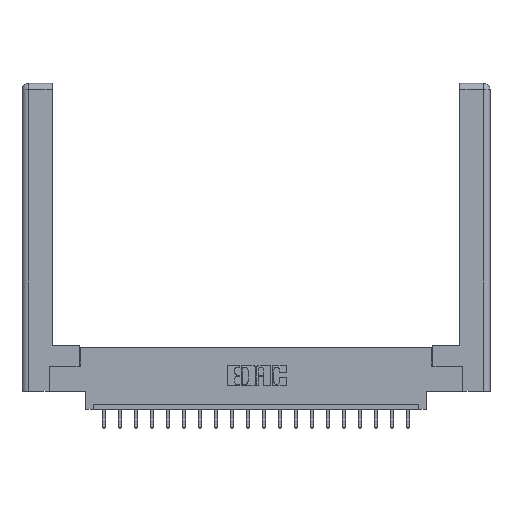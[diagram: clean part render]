
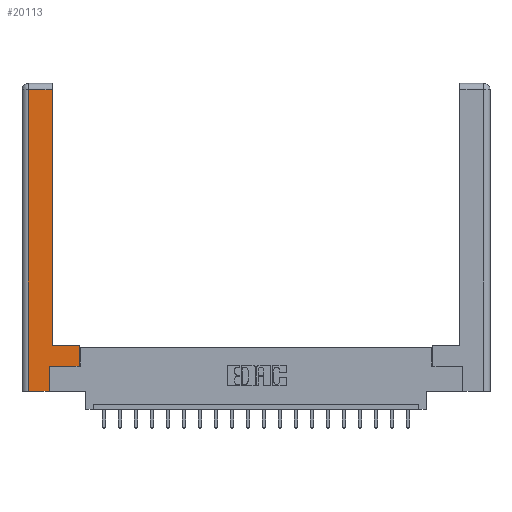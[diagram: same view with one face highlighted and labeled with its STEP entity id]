
A CAD part, top view. The second image highlights one B-rep face of the part: STEP entity #20113.
In plain terms, the highlighted planar face has unit normal (0, 0, 1).
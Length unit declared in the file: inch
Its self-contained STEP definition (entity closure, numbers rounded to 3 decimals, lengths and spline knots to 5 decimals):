
#619 = LINE ( 'NONE', #10233, #16537 ) ;
#1052 = ORIENTED_EDGE ( 'NONE', *, *, #16412, .T. ) ;
#1125 = VERTEX_POINT ( 'NONE', #10306 ) ;
#1255 = LINE ( 'NONE', #3558, #9013 ) ;
#1774 = LINE ( 'NONE', #10277, #2007 ) ;
#1930 = DIRECTION ( 'NONE',  ( 0., 1., 0. ) ) ;
#1994 = CARTESIAN_POINT ( 'NONE',  ( 0.0615, 2.94, 0. ) ) ;
#2007 = VECTOR ( 'NONE', #18453, 39.37008 ) ;
#2178 = EDGE_CURVE ( 'NONE', #15782, #13616, #1774, .T. ) ;
#2223 = ORIENTED_EDGE ( 'NONE', *, *, #10194, .T. ) ;
#2289 = CARTESIAN_POINT ( 'NONE',  ( 0.565, 0.245, 0. ) ) ;
#2512 = VECTOR ( 'NONE', #12896, 39.37008 ) ;
#3025 = DIRECTION ( 'NONE',  ( 0., 0., -1. ) ) ;
#3085 = EDGE_LOOP ( 'NONE', ( #16549, #2223, #18322, #14330, #16778, #1052, #13629, #8662 ) ) ;
#3558 = CARTESIAN_POINT ( 'NONE',  ( 0.295, 0.45, 0. ) ) ;
#3946 = DIRECTION ( 'NONE',  ( 1., 0., 0. ) ) ;
#4752 = CARTESIAN_POINT ( 'NONE',  ( 0.0615, 0., 0. ) ) ;
#5278 = CARTESIAN_POINT ( 'NONE',  ( 0.265, 0., 0. ) ) ;
#6030 = EDGE_CURVE ( 'NONE', #6105, #14938, #9864, .T. ) ;
#6105 = VERTEX_POINT ( 'NONE', #5278 ) ;
#6182 = EDGE_CURVE ( 'NONE', #7716, #6105, #619, .T. ) ;
#7032 = LINE ( 'NONE', #17950, #18241 ) ;
#7328 = CARTESIAN_POINT ( 'NONE',  ( 0.0615, 2.94, 0. ) ) ;
#7577 = EDGE_CURVE ( 'NONE', #14143, #1125, #7032, .T. ) ;
#7716 = VERTEX_POINT ( 'NONE', #18553 ) ;
#8306 = DIRECTION ( 'NONE',  ( 0., 1., 0. ) ) ;
#8662 = ORIENTED_EDGE ( 'NONE', *, *, #15277, .T. ) ;
#8668 = FACE_OUTER_BOUND ( 'NONE', #3085, .T. ) ;
#9013 = VECTOR ( 'NONE', #19487, 39.37008 ) ;
#9198 = LINE ( 'NONE', #18119, #13186 ) ;
#9386 = EDGE_CURVE ( 'NONE', #11728, #7716, #14218, .T. ) ;
#9810 = CARTESIAN_POINT ( 'NONE',  ( 0.265, 0.245, 0. ) ) ;
#9864 = LINE ( 'NONE', #9810, #18319 ) ;
#10194 = EDGE_CURVE ( 'NONE', #13616, #11728, #15916, .T. ) ;
#10233 = CARTESIAN_POINT ( 'NONE',  ( 0.265, 0., 0. ) ) ;
#10277 = CARTESIAN_POINT ( 'NONE',  ( 0.295, 3., 0. ) ) ;
#10306 = CARTESIAN_POINT ( 'NONE',  ( 0.565, 0.45, 0. ) ) ;
#10477 = VECTOR ( 'NONE', #13468, 39.37008 ) ;
#10992 = CARTESIAN_POINT ( 'NONE',  ( 0., 0., 0. ) ) ;
#11728 = VERTEX_POINT ( 'NONE', #1994 ) ;
#11969 = CARTESIAN_POINT ( 'NONE',  ( 0.295, 2.94, 0. ) ) ;
#12896 = DIRECTION ( 'NONE',  ( 0., -1., 0. ) ) ;
#13186 = VECTOR ( 'NONE', #18045, 39.37008 ) ;
#13468 = DIRECTION ( 'NONE',  ( -1., 0., 0. ) ) ;
#13616 = VERTEX_POINT ( 'NONE', #11969 ) ;
#13629 = ORIENTED_EDGE ( 'NONE', *, *, #7577, .T. ) ;
#14027 = AXIS2_PLACEMENT_3D ( 'NONE', #10992, #3025, #17436 ) ;
#14143 = VERTEX_POINT ( 'NONE', #2289 ) ;
#14218 = LINE ( 'NONE', #4752, #2512 ) ;
#14330 = ORIENTED_EDGE ( 'NONE', *, *, #6182, .T. ) ;
#14938 = VERTEX_POINT ( 'NONE', #15353 ) ;
#15277 = EDGE_CURVE ( 'NONE', #1125, #15782, #1255, .T. ) ;
#15353 = CARTESIAN_POINT ( 'NONE',  ( 0.265, 0.245, 0. ) ) ;
#15634 = PLANE ( 'NONE',  #14027 ) ;
#15782 = VERTEX_POINT ( 'NONE', #16459 ) ;
#15916 = LINE ( 'NONE', #7328, #10477 ) ;
#16412 = EDGE_CURVE ( 'NONE', #14938, #14143, #9198, .T. ) ;
#16459 = CARTESIAN_POINT ( 'NONE',  ( 0.295, 0.45, 0. ) ) ;
#16537 = VECTOR ( 'NONE', #3946, 39.37008 ) ;
#16549 = ORIENTED_EDGE ( 'NONE', *, *, #2178, .T. ) ;
#16778 = ORIENTED_EDGE ( 'NONE', *, *, #6030, .T. ) ;
#17436 = DIRECTION ( 'NONE',  ( -1., 0., 0. ) ) ;
#17950 = CARTESIAN_POINT ( 'NONE',  ( 0.565, 0.45, 0. ) ) ;
#18045 = DIRECTION ( 'NONE',  ( 1., 0., 0. ) ) ;
#18119 = CARTESIAN_POINT ( 'NONE',  ( 0.565, 0.245, 0. ) ) ;
#18241 = VECTOR ( 'NONE', #8306, 39.37008 ) ;
#18319 = VECTOR ( 'NONE', #1930, 39.37008 ) ;
#18322 = ORIENTED_EDGE ( 'NONE', *, *, #9386, .T. ) ;
#18453 = DIRECTION ( 'NONE',  ( 0., 1., 0. ) ) ;
#18553 = CARTESIAN_POINT ( 'NONE',  ( 0.0615, 0., 0. ) ) ;
#19487 = DIRECTION ( 'NONE',  ( -1., 0., 0. ) ) ;
#20113 = ADVANCED_FACE ( 'NONE', ( #8668 ), #15634, .F. ) ;
